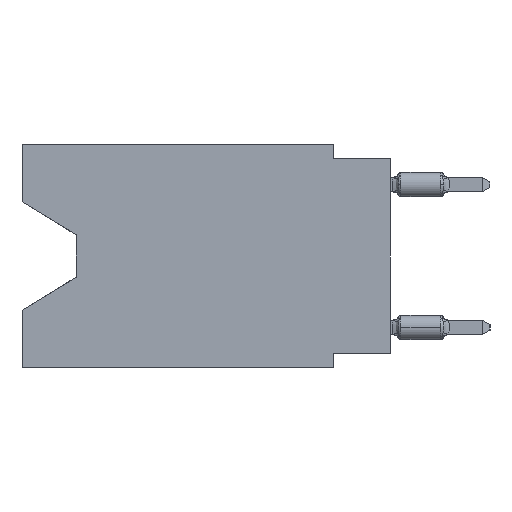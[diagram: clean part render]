
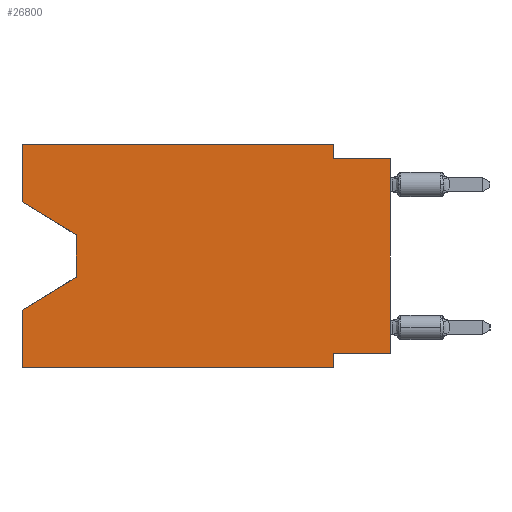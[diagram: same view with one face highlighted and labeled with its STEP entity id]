
A CAD part, left-side view. The second image highlights one B-rep face of the part: STEP entity #26800.
In plain terms, the highlighted planar face has unit normal (-1, 0, 0).
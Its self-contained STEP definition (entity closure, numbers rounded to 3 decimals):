
#169 = AXIS2_PLACEMENT_3D ( 'NONE', #24495, #2356, #24000 ) ;
#412 = CARTESIAN_POINT ( 'NONE',  ( 0., 16.383, -2.546 ) ) ;
#897 = DIRECTION ( 'NONE',  ( 0., 0., 1. ) ) ;
#1038 = VECTOR ( 'NONE', #43096, 1000. ) ;
#1107 = LINE ( 'NONE', #31882, #46744 ) ;
#1585 = CARTESIAN_POINT ( 'NONE',  ( 0., 16.383, 0. ) ) ;
#2089 = LINE ( 'NONE', #1585, #8771 ) ;
#2199 = LINE ( 'NONE', #24790, #36675 ) ;
#2356 = DIRECTION ( 'NONE',  ( 1., 0., 0. ) ) ;
#4307 = EDGE_CURVE ( 'NONE', #41590, #25958, #12863, .T. ) ;
#4623 = EDGE_CURVE ( 'NONE', #9695, #26537, #19316, .T. ) ;
#5578 = CARTESIAN_POINT ( 'NONE',  ( 0., 0., -0.635 ) ) ;
#7223 = ORIENTED_EDGE ( 'NONE', *, *, #4307, .F. ) ;
#7860 = ORIENTED_EDGE ( 'NONE', *, *, #32477, .F. ) ;
#8211 = CARTESIAN_POINT ( 'NONE',  ( 0., 16.383, 0. ) ) ;
#8771 = VECTOR ( 'NONE', #27851, 1000. ) ;
#8815 = EDGE_CURVE ( 'NONE', #13213, #41590, #47713, .T. ) ;
#8985 = CARTESIAN_POINT ( 'NONE',  ( 0., 2.54, 0. ) ) ;
#9652 = ORIENTED_EDGE ( 'NONE', *, *, #40835, .F. ) ;
#9695 = VERTEX_POINT ( 'NONE', #45835 ) ;
#9798 = VECTOR ( 'NONE', #20140, 1000. ) ;
#10578 = CARTESIAN_POINT ( 'NONE',  ( 0., 0., -9.271 ) ) ;
#11399 = FACE_OUTER_BOUND ( 'NONE', #40623, .T. ) ;
#11544 = CARTESIAN_POINT ( 'NONE',  ( 0., 0., -0.635 ) ) ;
#11816 = CARTESIAN_POINT ( 'NONE',  ( 0., 13.97, -5.893 ) ) ;
#12363 = CARTESIAN_POINT ( 'NONE',  ( 0., 2.54, -9.906 ) ) ;
#12863 = LINE ( 'NONE', #12363, #9798 ) ;
#12967 = CARTESIAN_POINT ( 'NONE',  ( 0., 2.54, 0. ) ) ;
#13213 = VERTEX_POINT ( 'NONE', #10578 ) ;
#13998 = EDGE_CURVE ( 'NONE', #32150, #20687, #36845, .T. ) ;
#15551 = VERTEX_POINT ( 'NONE', #35652 ) ;
#16670 = CARTESIAN_POINT ( 'NONE',  ( 0., 2.54, -9.271 ) ) ;
#16965 = ORIENTED_EDGE ( 'NONE', *, *, #4623, .F. ) ;
#17108 = VERTEX_POINT ( 'NONE', #35223 ) ;
#17327 = EDGE_CURVE ( 'NONE', #20687, #41372, #22564, .T. ) ;
#17945 = EDGE_CURVE ( 'NONE', #20880, #38206, #2089, .T. ) ;
#18402 = EDGE_CURVE ( 'NONE', #13213, #26537, #2199, .T. ) ;
#19316 = LINE ( 'NONE', #11544, #46965 ) ;
#19431 = ORIENTED_EDGE ( 'NONE', *, *, #8815, .F. ) ;
#19996 = ORIENTED_EDGE ( 'NONE', *, *, #30072, .F. ) ;
#20140 = DIRECTION ( 'NONE',  ( 0., 0., -1. ) ) ;
#20687 = VERTEX_POINT ( 'NONE', #34957 ) ;
#20880 = VERTEX_POINT ( 'NONE', #44656 ) ;
#21321 = CARTESIAN_POINT ( 'NONE',  ( 0., 13.97, -5.893 ) ) ;
#22564 = LINE ( 'NONE', #37348, #26557 ) ;
#23383 = CARTESIAN_POINT ( 'NONE',  ( 0., 16.383, 0. ) ) ;
#23647 = LINE ( 'NONE', #23383, #26797 ) ;
#24000 = DIRECTION ( 'NONE',  ( 0., 0., -1. ) ) ;
#24495 = CARTESIAN_POINT ( 'NONE',  ( 0., 16.383, 0. ) ) ;
#24790 = CARTESIAN_POINT ( 'NONE',  ( 0., 0., 0. ) ) ;
#25448 = LINE ( 'NONE', #21321, #36644 ) ;
#25958 = VERTEX_POINT ( 'NONE', #26329 ) ;
#26231 = DIRECTION ( 'NONE',  ( 0., 0., -1. ) ) ;
#26329 = CARTESIAN_POINT ( 'NONE',  ( 0., 2.54, -9.906 ) ) ;
#26364 = ORIENTED_EDGE ( 'NONE', *, *, #13998, .T. ) ;
#26483 = CARTESIAN_POINT ( 'NONE',  ( 0., 16.383, -2.546 ) ) ;
#26537 = VERTEX_POINT ( 'NONE', #5578 ) ;
#26557 = VECTOR ( 'NONE', #26231, 1000. ) ;
#26797 = VECTOR ( 'NONE', #38168, 1000. ) ;
#26800 = ADVANCED_FACE ( 'NONE', ( #11399 ), #38552, .F. ) ;
#27038 = EDGE_CURVE ( 'NONE', #41372, #17108, #25448, .T. ) ;
#27178 = EDGE_CURVE ( 'NONE', #15551, #25958, #1107, .T. ) ;
#27258 = VECTOR ( 'NONE', #897, 1000. ) ;
#27851 = DIRECTION ( 'NONE',  ( 0., -1., 0. ) ) ;
#29821 = DIRECTION ( 'NONE',  ( 0., -0.855, -0.519 ) ) ;
#30072 = EDGE_CURVE ( 'NONE', #15551, #17108, #23647, .T. ) ;
#31882 = CARTESIAN_POINT ( 'NONE',  ( 0., 16.383, -9.906 ) ) ;
#32150 = VERTEX_POINT ( 'NONE', #26483 ) ;
#32477 = EDGE_CURVE ( 'NONE', #32150, #20880, #37822, .T. ) ;
#34109 = DIRECTION ( 'NONE',  ( 0., -1., 0. ) ) ;
#34803 = DIRECTION ( 'NONE',  ( 0., 0., -1. ) ) ;
#34957 = CARTESIAN_POINT ( 'NONE',  ( 0., 13.97, -4.013 ) ) ;
#35223 = CARTESIAN_POINT ( 'NONE',  ( 0., 16.383, -7.36 ) ) ;
#35652 = CARTESIAN_POINT ( 'NONE',  ( 0., 16.383, -9.906 ) ) ;
#36644 = VECTOR ( 'NONE', #40227, 1000. ) ;
#36675 = VECTOR ( 'NONE', #46416, 1000. ) ;
#36845 = LINE ( 'NONE', #412, #42719 ) ;
#37348 = CARTESIAN_POINT ( 'NONE',  ( 0., 13.97, -4.013 ) ) ;
#37822 = LINE ( 'NONE', #8211, #27258 ) ;
#38034 = ORIENTED_EDGE ( 'NONE', *, *, #27178, .T. ) ;
#38119 = ORIENTED_EDGE ( 'NONE', *, *, #18402, .T. ) ;
#38168 = DIRECTION ( 'NONE',  ( 0., 0., 1. ) ) ;
#38182 = LINE ( 'NONE', #12967, #39893 ) ;
#38206 = VERTEX_POINT ( 'NONE', #8985 ) ;
#38552 = PLANE ( 'NONE',  #169 ) ;
#39440 = CARTESIAN_POINT ( 'NONE',  ( 0., 0., -9.271 ) ) ;
#39893 = VECTOR ( 'NONE', #34803, 1000. ) ;
#40227 = DIRECTION ( 'NONE',  ( 0., 0.855, -0.519 ) ) ;
#40623 = EDGE_LOOP ( 'NONE', ( #26364, #40650, #43188, #19996, #38034, #7223, #19431, #38119, #16965, #9652, #47201, #7860 ) ) ;
#40650 = ORIENTED_EDGE ( 'NONE', *, *, #17327, .T. ) ;
#40835 = EDGE_CURVE ( 'NONE', #38206, #9695, #38182, .T. ) ;
#41372 = VERTEX_POINT ( 'NONE', #11816 ) ;
#41590 = VERTEX_POINT ( 'NONE', #16670 ) ;
#42719 = VECTOR ( 'NONE', #29821, 1000. ) ;
#43096 = DIRECTION ( 'NONE',  ( 0., 1., 0. ) ) ;
#43188 = ORIENTED_EDGE ( 'NONE', *, *, #27038, .T. ) ;
#44656 = CARTESIAN_POINT ( 'NONE',  ( 0., 16.383, 0. ) ) ;
#45781 = DIRECTION ( 'NONE',  ( 0., -1., 0. ) ) ;
#45835 = CARTESIAN_POINT ( 'NONE',  ( 0., 2.54, -0.635 ) ) ;
#46416 = DIRECTION ( 'NONE',  ( 0., 0., 1. ) ) ;
#46744 = VECTOR ( 'NONE', #45781, 1000. ) ;
#46965 = VECTOR ( 'NONE', #34109, 1000. ) ;
#47201 = ORIENTED_EDGE ( 'NONE', *, *, #17945, .F. ) ;
#47713 = LINE ( 'NONE', #39440, #1038 ) ;
